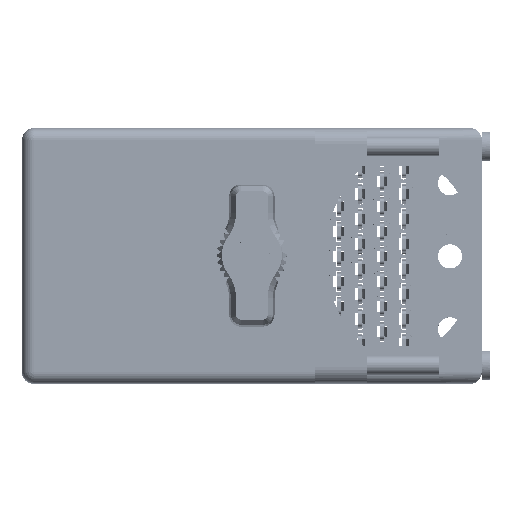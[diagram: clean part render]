
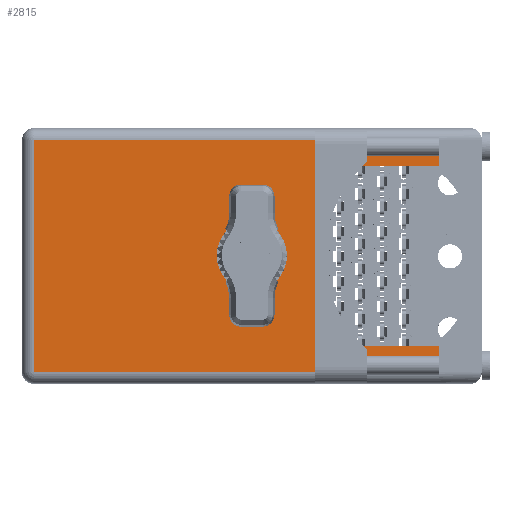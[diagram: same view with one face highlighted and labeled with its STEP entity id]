
A CAD part, top view. The second image highlights one B-rep face of the part: STEP entity #2815.
In plain terms, the highlighted face is planar.
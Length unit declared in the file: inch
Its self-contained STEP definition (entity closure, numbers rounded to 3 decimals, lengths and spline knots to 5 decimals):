
#13 = CARTESIAN_POINT ( 'NONE',  ( 0., 2.03, -1.53 ) ) ;
#748 = CARTESIAN_POINT ( 'NONE',  ( 2.499, 2.03, -1.53 ) ) ;
#1367 = CARTESIAN_POINT ( 'NONE',  ( 2.499, 2.03, -1.305 ) ) ;
#2815 = ADVANCED_FACE ( 'NONE', ( #10115, #52447 ), #92389, .T. ) ;
#3460 = DIRECTION ( 'NONE',  ( -1., 0., 0. ) ) ;
#3701 = VECTOR ( 'NONE', #32042, 39.37008 ) ;
#4270 = VERTEX_POINT ( 'NONE', #34646 ) ;
#6355 = LINE ( 'NONE', #90790, #3701 ) ;
#7364 = ORIENTED_EDGE ( 'NONE', *, *, #96183, .T. ) ;
#7896 = VECTOR ( 'NONE', #32816, 39.37008 ) ;
#10115 = FACE_OUTER_BOUND ( 'NONE', #41851, .T. ) ;
#10245 = VECTOR ( 'NONE', #3460, 39.37008 ) ;
#10608 = CIRCLE ( 'NONE', #49403, 0.17 ) ;
#15919 = VERTEX_POINT ( 'NONE', #76076 ) ;
#18426 = VECTOR ( 'NONE', #38330, 39.37008 ) ;
#23109 = CARTESIAN_POINT ( 'NONE',  ( 2.499, 2.03, -0.225 ) ) ;
#23128 = VERTEX_POINT ( 'NONE', #40802 ) ;
#24209 = EDGE_CURVE ( 'NONE', #4270, #15919, #10608, .T. ) ;
#24746 = VERTEX_POINT ( 'NONE', #55722 ) ;
#25260 = ORIENTED_EDGE ( 'NONE', *, *, #86854, .F. ) ;
#26445 = VERTEX_POINT ( 'NONE', #23109 ) ;
#26902 = EDGE_CURVE ( 'NONE', #24746, #42587, #31347, .T. ) ;
#27270 = VERTEX_POINT ( 'NONE', #82497 ) ;
#28761 = ORIENTED_EDGE ( 'NONE', *, *, #24209, .F. ) ;
#31347 = LINE ( 'NONE', #95835, #10245 ) ;
#31351 = EDGE_CURVE ( 'NONE', #35278, #77881, #52917, .T. ) ;
#31684 = DIRECTION ( 'NONE',  ( 0., 0., 1. ) ) ;
#32042 = DIRECTION ( 'NONE',  ( 0., 0., 1. ) ) ;
#32816 = DIRECTION ( 'NONE',  ( 1., 0., 0. ) ) ;
#32937 = EDGE_CURVE ( 'NONE', #15919, #4270, #90095, .T. ) ;
#33383 = ORIENTED_EDGE ( 'NONE', *, *, #94281, .F. ) ;
#34646 = CARTESIAN_POINT ( 'NONE',  ( 1.3775, 2.03, -0.595 ) ) ;
#35278 = VERTEX_POINT ( 'NONE', #61701 ) ;
#35331 = EDGE_LOOP ( 'NONE', ( #28761, #103385 ) ) ;
#36984 = ORIENTED_EDGE ( 'NONE', *, *, #49743, .T. ) ;
#37211 = CARTESIAN_POINT ( 'NONE',  ( 2.499, 2.03, -0.07 ) ) ;
#38330 = DIRECTION ( 'NONE',  ( 0., 0., -1. ) ) ;
#38875 = LINE ( 'NONE', #748, #108896 ) ;
#38950 = CARTESIAN_POINT ( 'NONE',  ( 2.499, 2.03, -0.07 ) ) ;
#40802 = CARTESIAN_POINT ( 'NONE',  ( 1.785, 2.03, -0.225 ) ) ;
#41261 = EDGE_CURVE ( 'NONE', #26445, #23128, #50051, .T. ) ;
#41719 = DIRECTION ( 'NONE',  ( 0., 0., 1. ) ) ;
#41851 = EDGE_LOOP ( 'NONE', ( #7364, #36984, #25260, #68083, #78036, #62353, #33383, #77389 ) ) ;
#42587 = VERTEX_POINT ( 'NONE', #50391 ) ;
#42917 = DIRECTION ( 'NONE',  ( 0., 1., 0. ) ) ;
#45706 = DIRECTION ( 'NONE',  ( 1., 0., 0. ) ) ;
#47246 = VERTEX_POINT ( 'NONE', #38950 ) ;
#47749 = DIRECTION ( 'NONE',  ( -1., 0., 0. ) ) ;
#48726 = CARTESIAN_POINT ( 'NONE',  ( 0.07, 2.03, -1.53 ) ) ;
#49403 = AXIS2_PLACEMENT_3D ( 'NONE', #83839, #49519, #100818 ) ;
#49519 = DIRECTION ( 'NONE',  ( 0., 1., 0. ) ) ;
#49743 = EDGE_CURVE ( 'NONE', #27270, #47246, #85514, .T. ) ;
#50051 = LINE ( 'NONE', #72109, #92315 ) ;
#50391 = CARTESIAN_POINT ( 'NONE',  ( 0.07, 2.03, -1.46 ) ) ;
#52447 = FACE_BOUND ( 'NONE', #35331, .T. ) ;
#52917 = LINE ( 'NONE', #109259, #7896 ) ;
#53250 = VECTOR ( 'NONE', #31684, 39.37008 ) ;
#54217 = AXIS2_PLACEMENT_3D ( 'NONE', #92290, #67934, #41719 ) ;
#55722 = CARTESIAN_POINT ( 'NONE',  ( 2.499, 2.03, -1.46 ) ) ;
#59933 = AXIS2_PLACEMENT_3D ( 'NONE', #13, #42917, #85340 ) ;
#61701 = CARTESIAN_POINT ( 'NONE',  ( 1.785, 2.03, -1.305 ) ) ;
#62353 = ORIENTED_EDGE ( 'NONE', *, *, #31351, .T. ) ;
#67934 = DIRECTION ( 'NONE',  ( 0., 1., 0. ) ) ;
#68083 = ORIENTED_EDGE ( 'NONE', *, *, #41261, .T. ) ;
#69973 = LINE ( 'NONE', #96676, #18426 ) ;
#72109 = CARTESIAN_POINT ( 'NONE',  ( 2.499, 2.03, -0.225 ) ) ;
#73692 = VECTOR ( 'NONE', #45706, 39.37008 ) ;
#75698 = LINE ( 'NONE', #48726, #53250 ) ;
#76076 = CARTESIAN_POINT ( 'NONE',  ( 1.3775, 2.03, -0.935 ) ) ;
#77389 = ORIENTED_EDGE ( 'NONE', *, *, #26902, .T. ) ;
#77881 = VERTEX_POINT ( 'NONE', #1367 ) ;
#78036 = ORIENTED_EDGE ( 'NONE', *, *, #104829, .T. ) ;
#82497 = CARTESIAN_POINT ( 'NONE',  ( 0.07, 2.03, -0.07 ) ) ;
#83839 = CARTESIAN_POINT ( 'NONE',  ( 1.3775, 2.03, -0.765 ) ) ;
#85340 = DIRECTION ( 'NONE',  ( 0., 0., 1. ) ) ;
#85514 = LINE ( 'NONE', #37211, #73692 ) ;
#86854 = EDGE_CURVE ( 'NONE', #26445, #47246, #38875, .T. ) ;
#90095 = CIRCLE ( 'NONE', #54217, 0.17 ) ;
#90790 = CARTESIAN_POINT ( 'NONE',  ( 2.499, 2.03, -1.53 ) ) ;
#92290 = CARTESIAN_POINT ( 'NONE',  ( 1.3775, 2.03, -0.765 ) ) ;
#92315 = VECTOR ( 'NONE', #47749, 39.37008 ) ;
#92389 = PLANE ( 'NONE',  #59933 ) ;
#94281 = EDGE_CURVE ( 'NONE', #24746, #77881, #6355, .T. ) ;
#95835 = CARTESIAN_POINT ( 'NONE',  ( 0., 2.03, -1.46 ) ) ;
#96183 = EDGE_CURVE ( 'NONE', #42587, #27270, #75698, .T. ) ;
#96676 = CARTESIAN_POINT ( 'NONE',  ( 1.785, 2.03, -1.305 ) ) ;
#100818 = DIRECTION ( 'NONE',  ( 0., 0., 1. ) ) ;
#102714 = DIRECTION ( 'NONE',  ( 0., 0., 1. ) ) ;
#103385 = ORIENTED_EDGE ( 'NONE', *, *, #32937, .F. ) ;
#104829 = EDGE_CURVE ( 'NONE', #23128, #35278, #69973, .T. ) ;
#108896 = VECTOR ( 'NONE', #102714, 39.37008 ) ;
#109259 = CARTESIAN_POINT ( 'NONE',  ( 2.499, 2.03, -1.305 ) ) ;
